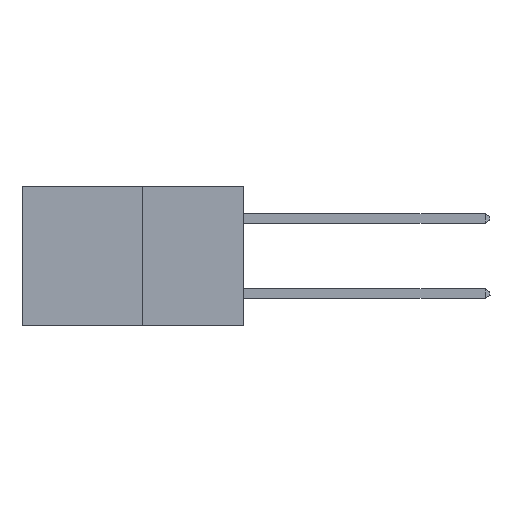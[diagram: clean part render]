
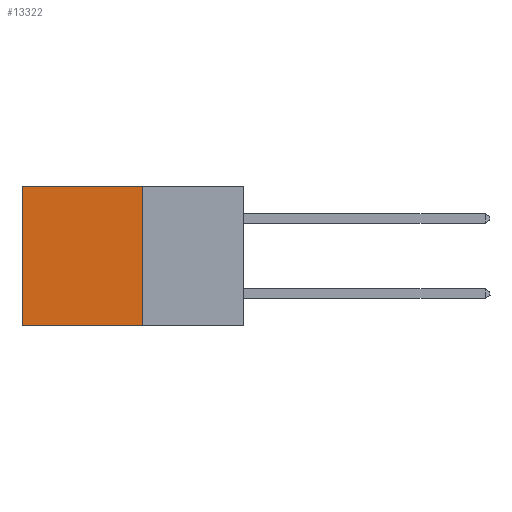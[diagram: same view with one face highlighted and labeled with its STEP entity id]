
A CAD part, left-side view. The second image highlights one B-rep face of the part: STEP entity #13322.
In plain terms, the highlighted planar face has unit normal (-1, 0, 0).
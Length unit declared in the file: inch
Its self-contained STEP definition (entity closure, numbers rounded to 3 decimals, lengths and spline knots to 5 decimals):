
#344 = VECTOR ( 'NONE', #2040, 39.37008 ) ;
#875 = DIRECTION ( 'NONE',  ( 1., 0., 0. ) ) ;
#924 = LINE ( 'NONE', #5471, #344 ) ;
#1952 = CARTESIAN_POINT ( 'NONE',  ( 0.277, 0.27, 0. ) ) ;
#2040 = DIRECTION ( 'NONE',  ( 0., 1., 0. ) ) ;
#2920 = CARTESIAN_POINT ( 'NONE',  ( 0.277, 0.59, -0.37 ) ) ;
#2924 = EDGE_LOOP ( 'NONE', ( #15514, #4601, #17743, #10462 ) ) ;
#4601 = ORIENTED_EDGE ( 'NONE', *, *, #10456, .F. ) ;
#5187 = CARTESIAN_POINT ( 'NONE',  ( 0.277, 0.59, 0. ) ) ;
#5471 = CARTESIAN_POINT ( 'NONE',  ( 0.277, 0.27, -0.37 ) ) ;
#5694 = VERTEX_POINT ( 'NONE', #20467 ) ;
#6560 = LINE ( 'NONE', #18293, #19785 ) ;
#7080 = VERTEX_POINT ( 'NONE', #5187 ) ;
#8098 = AXIS2_PLACEMENT_3D ( 'NONE', #11356, #875, #13100 ) ;
#8763 = DIRECTION ( 'NONE',  ( 0., 0., -1. ) ) ;
#10456 = EDGE_CURVE ( 'NONE', #5694, #21106, #924, .T. ) ;
#10462 = ORIENTED_EDGE ( 'NONE', *, *, #13345, .T. ) ;
#10829 = CARTESIAN_POINT ( 'NONE',  ( 0.277, 0.59, -0.37 ) ) ;
#11356 = CARTESIAN_POINT ( 'NONE',  ( 0.277, 0.27, -0.37 ) ) ;
#12063 = VECTOR ( 'NONE', #8763, 39.37008 ) ;
#12574 = DIRECTION ( 'NONE',  ( 0., 0., -1. ) ) ;
#13100 = DIRECTION ( 'NONE',  ( 0., 0., -1. ) ) ;
#13322 = ADVANCED_FACE ( 'NONE', ( #20340 ), #21635, .F. ) ;
#13345 = EDGE_CURVE ( 'NONE', #14280, #7080, #6560, .T. ) ;
#14280 = VERTEX_POINT ( 'NONE', #1952 ) ;
#15514 = ORIENTED_EDGE ( 'NONE', *, *, #21993, .T. ) ;
#16653 = LINE ( 'NONE', #20786, #12063 ) ;
#17743 = ORIENTED_EDGE ( 'NONE', *, *, #18587, .F. ) ;
#18293 = CARTESIAN_POINT ( 'NONE',  ( 0.277, 0.27, 0. ) ) ;
#18587 = EDGE_CURVE ( 'NONE', #14280, #5694, #16653, .T. ) ;
#19785 = VECTOR ( 'NONE', #20029, 39.37008 ) ;
#20029 = DIRECTION ( 'NONE',  ( 0., 1., 0. ) ) ;
#20340 = FACE_OUTER_BOUND ( 'NONE', #2924, .T. ) ;
#20467 = CARTESIAN_POINT ( 'NONE',  ( 0.277, 0.27, -0.37 ) ) ;
#20530 = VECTOR ( 'NONE', #12574, 39.37008 ) ;
#20786 = CARTESIAN_POINT ( 'NONE',  ( 0.277, 0.27, -0.37 ) ) ;
#21037 = LINE ( 'NONE', #10829, #20530 ) ;
#21106 = VERTEX_POINT ( 'NONE', #2920 ) ;
#21635 = PLANE ( 'NONE',  #8098 ) ;
#21993 = EDGE_CURVE ( 'NONE', #7080, #21106, #21037, .T. ) ;
